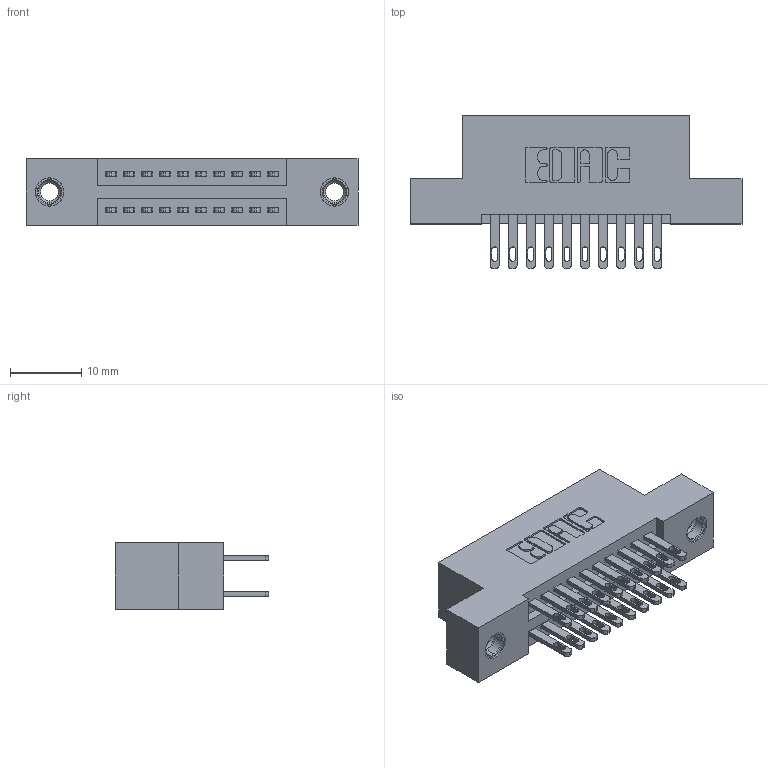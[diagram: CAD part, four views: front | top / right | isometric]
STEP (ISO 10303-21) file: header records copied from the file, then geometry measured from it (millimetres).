
FILE_DESCRIPTION (( 'STEP AP203' ), '1' );
FILE_NAME ('895-020-500-207.STEP', '2020-09-25T07:43:22', ( '' ), ( '' ), 'SwSTEP 2.0', 'SolidWorks 2020', '' );
FILE_SCHEMA (( 'CONFIG_CONTROL_DESIGN' ));
Length unit declared in the file: inch
Products named in the file (4): 345-250-001_345-250-005-103; 895-020-500-207; 345-292-001_345-293-100; 845 Part_Flush Mounting Lugs - 0.156 Dia-TI
Assembly tree (23 placements, depth 2):
  895-020-500-207
    845 Part_Flush Mounting Lugs - 0.156 Dia-TI
    345-292-001_345-293-100  x20
    345-250-001_345-250-005-103  x2
Bounding box: 46.61 x 21.51 x 9.4 mm (x, y, z)
Volume: 4278.2 mm3; surface area: 5936 mm2
Topology: 23 solids, 23 shells, 1106 faces, 3297 edges, 2190 vertices
Faces by surface type: plane 652, cylinder 438, cone 12, torus 4
Entity records: 13270 total; most frequent: CARTESIAN_POINT 2235, ORIENTED_EDGE 2162, DIRECTION 2039, EDGE_CURVE 1081, LINE 885, VECTOR 885, VERTEX_POINT 716, AXIS2_PLACEMENT_3D 577
